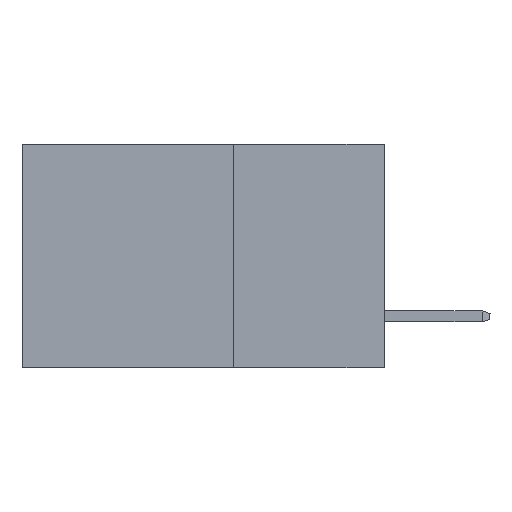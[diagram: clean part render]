
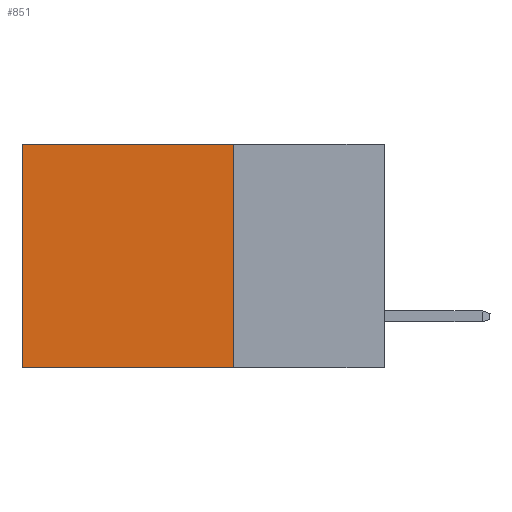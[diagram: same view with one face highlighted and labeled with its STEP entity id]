
A CAD part, left-side view. The second image highlights one B-rep face of the part: STEP entity #851.
In plain terms, the highlighted planar face has unit normal (-1, 0, 0).
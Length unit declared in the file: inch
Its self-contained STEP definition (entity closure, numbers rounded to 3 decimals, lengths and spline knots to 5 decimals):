
#49 = LINE ( 'NONE', #8365, #5442 ) ;
#791 = DIRECTION ( 'NONE',  ( 0., 1., 0. ) ) ;
#851 = ADVANCED_FACE ( 'NONE', ( #17610 ), #9173, .F. ) ;
#878 = EDGE_CURVE ( 'NONE', #3554, #4565, #49, .T. ) ;
#1623 = EDGE_LOOP ( 'NONE', ( #4977, #1653, #9114, #7734 ) ) ;
#1653 = ORIENTED_EDGE ( 'NONE', *, *, #13926, .F. ) ;
#2229 = DIRECTION ( 'NONE',  ( 1., 0., 0. ) ) ;
#2239 = VERTEX_POINT ( 'NONE', #5495 ) ;
#2386 = EDGE_CURVE ( 'NONE', #3554, #2239, #16025, .T. ) ;
#2859 = DIRECTION ( 'NONE',  ( 0., 0., -1. ) ) ;
#3537 = CARTESIAN_POINT ( 'NONE',  ( 0.298, 0.6, -0.37 ) ) ;
#3554 = VERTEX_POINT ( 'NONE', #11485 ) ;
#3564 = CARTESIAN_POINT ( 'NONE',  ( 0.298, 0.25, -0.37 ) ) ;
#3932 = CARTESIAN_POINT ( 'NONE',  ( 0.298, 0.6, 0. ) ) ;
#4220 = VECTOR ( 'NONE', #13865, 39.37008 ) ;
#4565 = VERTEX_POINT ( 'NONE', #4992 ) ;
#4977 = ORIENTED_EDGE ( 'NONE', *, *, #10701, .T. ) ;
#4992 = CARTESIAN_POINT ( 'NONE',  ( 0.298, 0.6, 0. ) ) ;
#5442 = VECTOR ( 'NONE', #17183, 39.37008 ) ;
#5495 = CARTESIAN_POINT ( 'NONE',  ( 0.298, 0.25, -0.37 ) ) ;
#6374 = DIRECTION ( 'NONE',  ( 0., 0., -1. ) ) ;
#7734 = ORIENTED_EDGE ( 'NONE', *, *, #878, .T. ) ;
#7933 = LINE ( 'NONE', #3932, #4220 ) ;
#8365 = CARTESIAN_POINT ( 'NONE',  ( 0.298, 0.25, 0. ) ) ;
#9114 = ORIENTED_EDGE ( 'NONE', *, *, #2386, .F. ) ;
#9173 = PLANE ( 'NONE',  #10664 ) ;
#9668 = VECTOR ( 'NONE', #2859, 39.37008 ) ;
#10664 = AXIS2_PLACEMENT_3D ( 'NONE', #13467, #2229, #6374 ) ;
#10701 = EDGE_CURVE ( 'NONE', #4565, #12654, #7933, .T. ) ;
#11450 = LINE ( 'NONE', #3564, #13418 ) ;
#11485 = CARTESIAN_POINT ( 'NONE',  ( 0.298, 0.25, 0. ) ) ;
#12654 = VERTEX_POINT ( 'NONE', #3537 ) ;
#13418 = VECTOR ( 'NONE', #791, 39.37008 ) ;
#13467 = CARTESIAN_POINT ( 'NONE',  ( 0.298, 0.25, 0. ) ) ;
#13865 = DIRECTION ( 'NONE',  ( 0., 0., -1. ) ) ;
#13926 = EDGE_CURVE ( 'NONE', #2239, #12654, #11450, .T. ) ;
#16025 = LINE ( 'NONE', #17056, #9668 ) ;
#17056 = CARTESIAN_POINT ( 'NONE',  ( 0.298, 0.25, 0. ) ) ;
#17183 = DIRECTION ( 'NONE',  ( 0., 1., 0. ) ) ;
#17610 = FACE_OUTER_BOUND ( 'NONE', #1623, .T. ) ;
